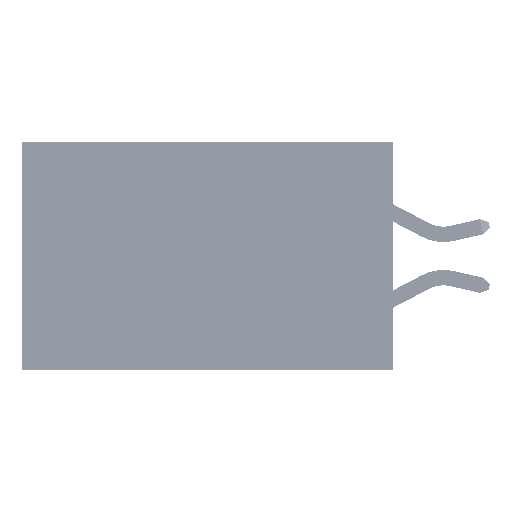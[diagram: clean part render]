
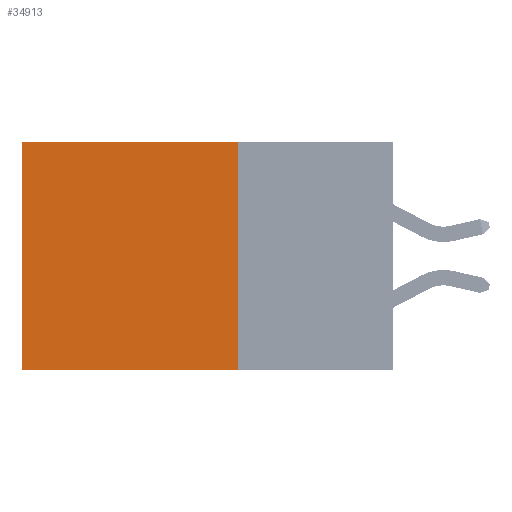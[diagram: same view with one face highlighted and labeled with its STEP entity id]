
A CAD part, left-side view. The second image highlights one B-rep face of the part: STEP entity #34913.
In plain terms, the highlighted planar face has unit normal (-1, 0, 0).
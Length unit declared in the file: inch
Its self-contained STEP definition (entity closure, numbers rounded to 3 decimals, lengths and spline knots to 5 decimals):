
#762 = DIRECTION ( 'NONE',  ( 0., 0., -1. ) ) ;
#1033 = CARTESIAN_POINT ( 'NONE',  ( 0.2875, 0.25, 0. ) ) ;
#1179 = EDGE_CURVE ( 'NONE', #49688, #33484, #10529, .T. ) ;
#1811 = DIRECTION ( 'NONE',  ( 0., 1., 0. ) ) ;
#1881 = LINE ( 'NONE', #27023, #42781 ) ;
#2560 = DIRECTION ( 'NONE',  ( 0., 0., -1. ) ) ;
#5739 = DIRECTION ( 'NONE',  ( 0., 1., 0. ) ) ;
#7959 = VECTOR ( 'NONE', #2560, 39.37008 ) ;
#8970 = ORIENTED_EDGE ( 'NONE', *, *, #29118, .F. ) ;
#10529 = LINE ( 'NONE', #46396, #7959 ) ;
#13639 = CARTESIAN_POINT ( 'NONE',  ( 0.2875, 0.25, 0. ) ) ;
#13973 = ORIENTED_EDGE ( 'NONE', *, *, #28193, .T. ) ;
#14535 = VERTEX_POINT ( 'NONE', #13639 ) ;
#15166 = EDGE_CURVE ( 'NONE', #14535, #15636, #1881, .T. ) ;
#15636 = VERTEX_POINT ( 'NONE', #34663 ) ;
#17237 = DIRECTION ( 'NONE',  ( 1., 0., 0. ) ) ;
#17494 = VECTOR ( 'NONE', #5739, 39.37008 ) ;
#17753 = PLANE ( 'NONE',  #50953 ) ;
#21495 = LINE ( 'NONE', #29976, #45563 ) ;
#24881 = LINE ( 'NONE', #49837, #17494 ) ;
#27023 = CARTESIAN_POINT ( 'NONE',  ( 0.2875, 0.25, 0. ) ) ;
#28193 = EDGE_CURVE ( 'NONE', #14535, #49688, #24881, .T. ) ;
#29118 = EDGE_CURVE ( 'NONE', #15636, #33484, #21495, .T. ) ;
#29976 = CARTESIAN_POINT ( 'NONE',  ( 0.2875, 0.25, -0.37 ) ) ;
#31489 = ORIENTED_EDGE ( 'NONE', *, *, #15166, .F. ) ;
#33484 = VERTEX_POINT ( 'NONE', #44857 ) ;
#33682 = FACE_OUTER_BOUND ( 'NONE', #42415, .T. ) ;
#34663 = CARTESIAN_POINT ( 'NONE',  ( 0.2875, 0.25, -0.37 ) ) ;
#34913 = ADVANCED_FACE ( 'NONE', ( #33682 ), #17753, .F. ) ;
#37320 = ORIENTED_EDGE ( 'NONE', *, *, #1179, .T. ) ;
#39788 = DIRECTION ( 'NONE',  ( 0., 0., -1. ) ) ;
#42415 = EDGE_LOOP ( 'NONE', ( #37320, #8970, #31489, #13973 ) ) ;
#42781 = VECTOR ( 'NONE', #39788, 39.37008 ) ;
#44857 = CARTESIAN_POINT ( 'NONE',  ( 0.2875, 0.6, -0.37 ) ) ;
#45291 = CARTESIAN_POINT ( 'NONE',  ( 0.2875, 0.6, 0. ) ) ;
#45563 = VECTOR ( 'NONE', #1811, 39.37008 ) ;
#46396 = CARTESIAN_POINT ( 'NONE',  ( 0.2875, 0.6, 0. ) ) ;
#49688 = VERTEX_POINT ( 'NONE', #45291 ) ;
#49837 = CARTESIAN_POINT ( 'NONE',  ( 0.2875, 0.25, 0. ) ) ;
#50953 = AXIS2_PLACEMENT_3D ( 'NONE', #1033, #17237, #762 ) ;
